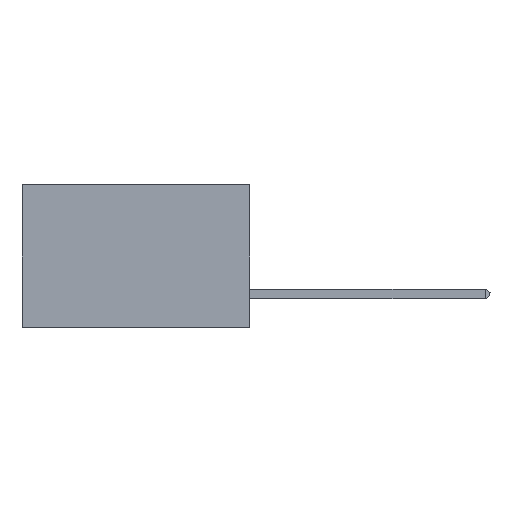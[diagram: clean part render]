
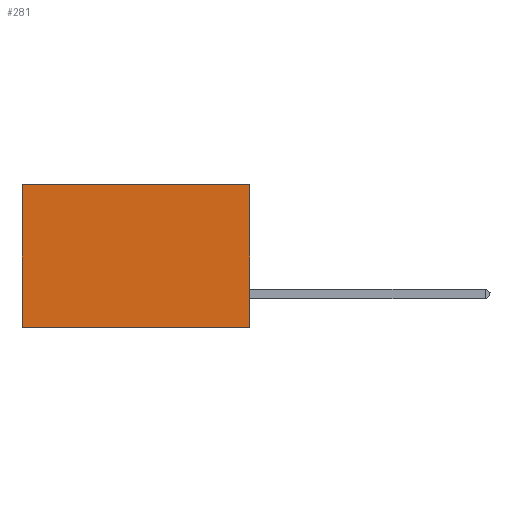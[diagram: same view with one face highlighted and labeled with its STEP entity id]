
A CAD part, left-side view. The second image highlights one B-rep face of the part: STEP entity #281.
In plain terms, the highlighted planar face has unit normal (-1, 0, 0).
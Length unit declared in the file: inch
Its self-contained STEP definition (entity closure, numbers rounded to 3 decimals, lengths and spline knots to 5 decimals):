
#281 = ADVANCED_FACE ( 'NONE', ( #17640 ), #16612, .F. ) ;
#776 = CARTESIAN_POINT ( 'NONE',  ( 0.2875, 0., -0.375 ) ) ;
#1466 = CARTESIAN_POINT ( 'NONE',  ( 0.2875, 0., -0.375 ) ) ;
#1530 = CARTESIAN_POINT ( 'NONE',  ( 0.2875, 0., 0. ) ) ;
#1916 = EDGE_CURVE ( 'NONE', #10965, #18894, #18071, .T. ) ;
#2042 = EDGE_CURVE ( 'NONE', #12868, #10965, #6122, .T. ) ;
#2231 = EDGE_CURVE ( 'NONE', #12868, #17581, #8383, .T. ) ;
#3395 = DIRECTION ( 'NONE',  ( 0., 1., 0. ) ) ;
#3822 = CARTESIAN_POINT ( 'NONE',  ( 0.2875, 0., -0.375 ) ) ;
#4101 = VECTOR ( 'NONE', #3395, 39.37008 ) ;
#4125 = VECTOR ( 'NONE', #10332, 39.37008 ) ;
#4458 = CARTESIAN_POINT ( 'NONE',  ( 0.2875, 0., 0. ) ) ;
#4661 = DIRECTION ( 'NONE',  ( 0., 0., -1. ) ) ;
#5568 = DIRECTION ( 'NONE',  ( 0., 0., -1. ) ) ;
#6122 = LINE ( 'NONE', #1466, #10621 ) ;
#7021 = EDGE_CURVE ( 'NONE', #17581, #18894, #18340, .T. ) ;
#8383 = LINE ( 'NONE', #1530, #4101 ) ;
#9731 = EDGE_LOOP ( 'NONE', ( #17084, #12059, #14103, #18864 ) ) ;
#10332 = DIRECTION ( 'NONE',  ( 0., 1., 0. ) ) ;
#10621 = VECTOR ( 'NONE', #4661, 39.37008 ) ;
#10965 = VERTEX_POINT ( 'NONE', #776 ) ;
#12059 = ORIENTED_EDGE ( 'NONE', *, *, #1916, .F. ) ;
#12542 = AXIS2_PLACEMENT_3D ( 'NONE', #13710, #13978, #13900 ) ;
#12868 = VERTEX_POINT ( 'NONE', #4458 ) ;
#13710 = CARTESIAN_POINT ( 'NONE',  ( 0.2875, 0., -0.375 ) ) ;
#13900 = DIRECTION ( 'NONE',  ( 0., 0., -1. ) ) ;
#13978 = DIRECTION ( 'NONE',  ( 1., 0., 0. ) ) ;
#14103 = ORIENTED_EDGE ( 'NONE', *, *, #2042, .F. ) ;
#15039 = CARTESIAN_POINT ( 'NONE',  ( 0.2875, 0.6, -0.375 ) ) ;
#16353 = VECTOR ( 'NONE', #5568, 39.37008 ) ;
#16612 = PLANE ( 'NONE',  #12542 ) ;
#17005 = CARTESIAN_POINT ( 'NONE',  ( 0.2875, 0.6, -0.375 ) ) ;
#17084 = ORIENTED_EDGE ( 'NONE', *, *, #7021, .T. ) ;
#17581 = VERTEX_POINT ( 'NONE', #20021 ) ;
#17640 = FACE_OUTER_BOUND ( 'NONE', #9731, .T. ) ;
#18071 = LINE ( 'NONE', #3822, #4125 ) ;
#18340 = LINE ( 'NONE', #15039, #16353 ) ;
#18864 = ORIENTED_EDGE ( 'NONE', *, *, #2231, .T. ) ;
#18894 = VERTEX_POINT ( 'NONE', #17005 ) ;
#20021 = CARTESIAN_POINT ( 'NONE',  ( 0.2875, 0.6, 0. ) ) ;
